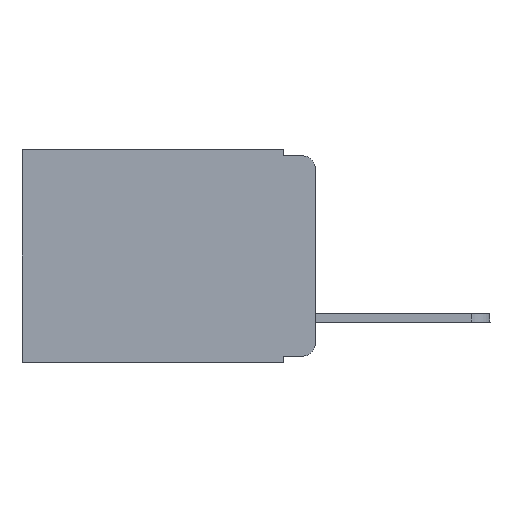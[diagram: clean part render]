
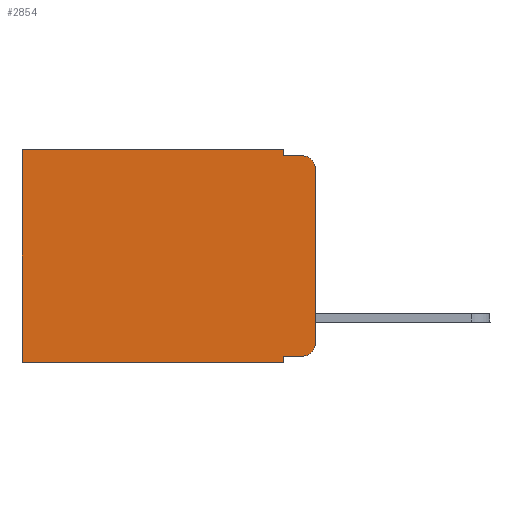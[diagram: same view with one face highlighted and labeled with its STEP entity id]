
A CAD part, left-side view. The second image highlights one B-rep face of the part: STEP entity #2854.
In plain terms, the highlighted planar face has unit normal (-1, 0, 0).
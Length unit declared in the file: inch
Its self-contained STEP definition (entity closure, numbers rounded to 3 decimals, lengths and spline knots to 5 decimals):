
#84 = EDGE_CURVE ( 'NONE', #10964, #11012, #10636, .T. ) ;
#228 = CARTESIAN_POINT ( 'NONE',  ( 0.298, 0., 0. ) ) ;
#266 = DIRECTION ( 'NONE',  ( -1., 0., 0. ) ) ;
#531 = CARTESIAN_POINT ( 'NONE',  ( 0.298, 0., 0. ) ) ;
#586 = ORIENTED_EDGE ( 'NONE', *, *, #9810, .F. ) ;
#846 = VERTEX_POINT ( 'NONE', #11006 ) ;
#917 = CARTESIAN_POINT ( 'NONE',  ( 0.298, 0.473, 0. ) ) ;
#937 = VECTOR ( 'NONE', #9896, 39.37008 ) ;
#1129 = CARTESIAN_POINT ( 'NONE',  ( 0.298, 0.02, -0.313 ) ) ;
#1144 = VERTEX_POINT ( 'NONE', #2410 ) ;
#1160 = DIRECTION ( 'NONE',  ( 0., 0., -1. ) ) ;
#1163 = CARTESIAN_POINT ( 'NONE',  ( 0.298, 0.051, -0.01 ) ) ;
#1393 = LINE ( 'NONE', #9065, #3258 ) ;
#1442 = DIRECTION ( 'NONE',  ( 1., 0., 0. ) ) ;
#1525 = DIRECTION ( 'NONE',  ( 0., 0., -1. ) ) ;
#1562 = EDGE_LOOP ( 'NONE', ( #7119, #3013, #8078, #10097, #10677, #12382, #12551, #586, #1903, #10519 ) ) ;
#1826 = VERTEX_POINT ( 'NONE', #2816 ) ;
#1903 = ORIENTED_EDGE ( 'NONE', *, *, #10755, .T. ) ;
#2111 = CARTESIAN_POINT ( 'NONE',  ( 0.298, 0., 0. ) ) ;
#2145 = CARTESIAN_POINT ( 'NONE',  ( 0.298, 0.473, -0.343 ) ) ;
#2183 = LINE ( 'NONE', #5706, #8425 ) ;
#2410 = CARTESIAN_POINT ( 'NONE',  ( 0.298, 0.473, 0. ) ) ;
#2501 = DIRECTION ( 'NONE',  ( 0., -1., 0. ) ) ;
#2671 = VECTOR ( 'NONE', #2501, 39.37008 ) ;
#2816 = CARTESIAN_POINT ( 'NONE',  ( 0.298, 0.051, 0. ) ) ;
#2837 = VERTEX_POINT ( 'NONE', #9428 ) ;
#2854 = ADVANCED_FACE ( 'NONE', ( #7096 ), #5578, .F. ) ;
#3013 = ORIENTED_EDGE ( 'NONE', *, *, #9770, .T. ) ;
#3141 = DIRECTION ( 'NONE',  ( 0., 0., -1. ) ) ;
#3194 = VERTEX_POINT ( 'NONE', #7890 ) ;
#3258 = VECTOR ( 'NONE', #1160, 39.37008 ) ;
#3585 = VECTOR ( 'NONE', #7398, 39.37008 ) ;
#3711 = AXIS2_PLACEMENT_3D ( 'NONE', #1129, #266, #3141 ) ;
#4029 = CARTESIAN_POINT ( 'NONE',  ( 0.298, 0.02, -0.03 ) ) ;
#4133 = DIRECTION ( 'NONE',  ( 0., 0., -1. ) ) ;
#4843 = LINE ( 'NONE', #917, #11723 ) ;
#4900 = DIRECTION ( 'NONE',  ( 0., 0., -1. ) ) ;
#5338 = CIRCLE ( 'NONE', #7769, 0.02 ) ;
#5578 = PLANE ( 'NONE',  #7384 ) ;
#5706 = CARTESIAN_POINT ( 'NONE',  ( 0.298, 0.051, -0.01 ) ) ;
#5742 = DIRECTION ( 'NONE',  ( 0., -1., 0. ) ) ;
#5996 = CARTESIAN_POINT ( 'NONE',  ( 0.298, 0.051, -0.343 ) ) ;
#6122 = DIRECTION ( 'NONE',  ( 0., 1., 0. ) ) ;
#6253 = LINE ( 'NONE', #2111, #11245 ) ;
#6787 = EDGE_CURVE ( 'NONE', #1826, #9918, #1393, .T. ) ;
#7024 = LINE ( 'NONE', #8471, #2671 ) ;
#7096 = FACE_OUTER_BOUND ( 'NONE', #1562, .T. ) ;
#7119 = ORIENTED_EDGE ( 'NONE', *, *, #12797, .F. ) ;
#7384 = AXIS2_PLACEMENT_3D ( 'NONE', #531, #1442, #1525 ) ;
#7398 = DIRECTION ( 'NONE',  ( 0., 1., 0. ) ) ;
#7407 = CARTESIAN_POINT ( 'NONE',  ( 0.298, 0.02, -0.01 ) ) ;
#7769 = AXIS2_PLACEMENT_3D ( 'NONE', #4029, #11082, #10994 ) ;
#7782 = EDGE_CURVE ( 'NONE', #8351, #846, #8071, .T. ) ;
#7838 = VERTEX_POINT ( 'NONE', #7407 ) ;
#7890 = CARTESIAN_POINT ( 'NONE',  ( 0.298, 0., -0.03 ) ) ;
#7927 = CARTESIAN_POINT ( 'NONE',  ( 0.298, 0.051, 0. ) ) ;
#8071 = CIRCLE ( 'NONE', #3711, 0.02 ) ;
#8078 = ORIENTED_EDGE ( 'NONE', *, *, #10216, .F. ) ;
#8351 = VERTEX_POINT ( 'NONE', #12245 ) ;
#8425 = VECTOR ( 'NONE', #5742, 39.37008 ) ;
#8471 = CARTESIAN_POINT ( 'NONE',  ( 0.298, 0.051, -0.333 ) ) ;
#8526 = LINE ( 'NONE', #228, #9173 ) ;
#8743 = LINE ( 'NONE', #7927, #937 ) ;
#9065 = CARTESIAN_POINT ( 'NONE',  ( 0.298, 0.051, 0. ) ) ;
#9173 = VECTOR ( 'NONE', #4133, 39.37008 ) ;
#9422 = CARTESIAN_POINT ( 'NONE',  ( 0.298, 0., -0.343 ) ) ;
#9428 = CARTESIAN_POINT ( 'NONE',  ( 0.298, 0.051, -0.333 ) ) ;
#9770 = EDGE_CURVE ( 'NONE', #3194, #7838, #5338, .T. ) ;
#9810 = EDGE_CURVE ( 'NONE', #2837, #10964, #8743, .T. ) ;
#9896 = DIRECTION ( 'NONE',  ( 0., 0., -1. ) ) ;
#9918 = VERTEX_POINT ( 'NONE', #1163 ) ;
#10097 = ORIENTED_EDGE ( 'NONE', *, *, #6787, .F. ) ;
#10216 = EDGE_CURVE ( 'NONE', #9918, #7838, #2183, .T. ) ;
#10519 = ORIENTED_EDGE ( 'NONE', *, *, #7782, .T. ) ;
#10636 = LINE ( 'NONE', #9422, #3585 ) ;
#10677 = ORIENTED_EDGE ( 'NONE', *, *, #11067, .T. ) ;
#10755 = EDGE_CURVE ( 'NONE', #2837, #8351, #7024, .T. ) ;
#10928 = EDGE_CURVE ( 'NONE', #1144, #11012, #4843, .T. ) ;
#10964 = VERTEX_POINT ( 'NONE', #5996 ) ;
#10994 = DIRECTION ( 'NONE',  ( 0., 0., -1. ) ) ;
#11006 = CARTESIAN_POINT ( 'NONE',  ( 0.298, 0., -0.313 ) ) ;
#11012 = VERTEX_POINT ( 'NONE', #2145 ) ;
#11067 = EDGE_CURVE ( 'NONE', #1826, #1144, #6253, .T. ) ;
#11082 = DIRECTION ( 'NONE',  ( -1., 0., 0. ) ) ;
#11245 = VECTOR ( 'NONE', #6122, 39.37008 ) ;
#11723 = VECTOR ( 'NONE', #4900, 39.37008 ) ;
#12245 = CARTESIAN_POINT ( 'NONE',  ( 0.298, 0.02, -0.333 ) ) ;
#12382 = ORIENTED_EDGE ( 'NONE', *, *, #10928, .T. ) ;
#12551 = ORIENTED_EDGE ( 'NONE', *, *, #84, .F. ) ;
#12797 = EDGE_CURVE ( 'NONE', #3194, #846, #8526, .T. ) ;
